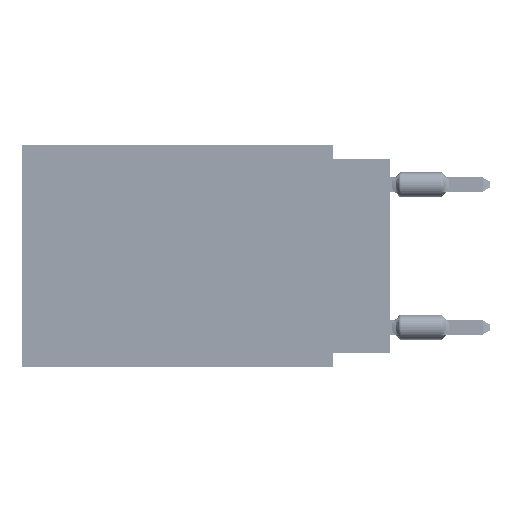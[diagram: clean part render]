
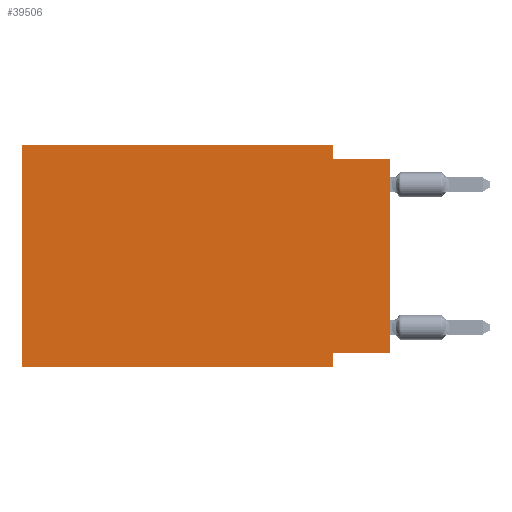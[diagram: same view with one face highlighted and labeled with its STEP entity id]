
A CAD part, left-side view. The second image highlights one B-rep face of the part: STEP entity #39506.
In plain terms, the highlighted planar face has unit normal (-1, 0, 0).
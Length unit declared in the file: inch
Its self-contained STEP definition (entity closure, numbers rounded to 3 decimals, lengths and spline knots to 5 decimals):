
#52 = ORIENTED_EDGE ( 'NONE', *, *, #19391, .F. ) ;
#125 = DIRECTION ( 'NONE',  ( 0., -1., 0. ) ) ;
#3661 = LINE ( 'NONE', #63159, #73262 ) ;
#3766 = CARTESIAN_POINT ( 'NONE',  ( 0., 0.1, -0.39 ) ) ;
#4742 = ORIENTED_EDGE ( 'NONE', *, *, #81338, .F. ) ;
#4808 = EDGE_LOOP ( 'NONE', ( #37551, #9426, #4742, #25082, #52, #56656, #25058, #45103 ) ) ;
#6551 = LINE ( 'NONE', #32664, #82076 ) ;
#8865 = VECTOR ( 'NONE', #70994, 39.37008 ) ;
#9426 = ORIENTED_EDGE ( 'NONE', *, *, #51864, .F. ) ;
#10950 = DIRECTION ( 'NONE',  ( 0., 0., -1. ) ) ;
#12824 = DIRECTION ( 'NONE',  ( 0., -1., 0. ) ) ;
#12857 = VECTOR ( 'NONE', #12824, 39.37008 ) ;
#14466 = VERTEX_POINT ( 'NONE', #17060 ) ;
#17060 = CARTESIAN_POINT ( 'NONE',  ( 0., 0.1, -0.025 ) ) ;
#17322 = CARTESIAN_POINT ( 'NONE',  ( 0., 0.1, -0.39 ) ) ;
#17599 = DIRECTION ( 'NONE',  ( 0., 0., -1. ) ) ;
#17921 = CARTESIAN_POINT ( 'NONE',  ( 0., 0.645, 0. ) ) ;
#17949 = VECTOR ( 'NONE', #71335, 39.37008 ) ;
#18405 = VERTEX_POINT ( 'NONE', #35603 ) ;
#19391 = EDGE_CURVE ( 'NONE', #18405, #36126, #3661, .T. ) ;
#21818 = FACE_OUTER_BOUND ( 'NONE', #4808, .T. ) ;
#22220 = CARTESIAN_POINT ( 'NONE',  ( 0., 0.645, 0. ) ) ;
#22279 = VECTOR ( 'NONE', #74169, 39.37008 ) ;
#23789 = DIRECTION ( 'NONE',  ( 1., 0., 0. ) ) ;
#24420 = CARTESIAN_POINT ( 'NONE',  ( 0., 0.1, 0. ) ) ;
#25058 = ORIENTED_EDGE ( 'NONE', *, *, #36834, .F. ) ;
#25082 = ORIENTED_EDGE ( 'NONE', *, *, #52332, .F. ) ;
#26493 = VECTOR ( 'NONE', #62937, 39.37008 ) ;
#31933 = CARTESIAN_POINT ( 'NONE',  ( 0., 0., -0.365 ) ) ;
#32664 = CARTESIAN_POINT ( 'NONE',  ( 0., 0.645, -0.39 ) ) ;
#32752 = VERTEX_POINT ( 'NONE', #67781 ) ;
#35136 = CARTESIAN_POINT ( 'NONE',  ( 0., 0.645, 0. ) ) ;
#35603 = CARTESIAN_POINT ( 'NONE',  ( 0., 0.645, -0.39 ) ) ;
#36126 = VERTEX_POINT ( 'NONE', #35136 ) ;
#36834 = EDGE_CURVE ( 'NONE', #72345, #54235, #74851, .T. ) ;
#37551 = ORIENTED_EDGE ( 'NONE', *, *, #62501, .T. ) ;
#39090 = EDGE_CURVE ( 'NONE', #45189, #72345, #48071, .T. ) ;
#39506 = ADVANCED_FACE ( 'NONE', ( #21818 ), #47973, .F. ) ;
#44523 = EDGE_CURVE ( 'NONE', #18405, #54235, #6551, .T. ) ;
#45103 = ORIENTED_EDGE ( 'NONE', *, *, #39090, .F. ) ;
#45189 = VERTEX_POINT ( 'NONE', #31933 ) ;
#45321 = LINE ( 'NONE', #17921, #8865 ) ;
#47973 = PLANE ( 'NONE',  #77065 ) ;
#48071 = LINE ( 'NONE', #68587, #22279 ) ;
#50905 = CARTESIAN_POINT ( 'NONE',  ( 0., 0., 0. ) ) ;
#51327 = LINE ( 'NONE', #50905, #26493 ) ;
#51374 = VERTEX_POINT ( 'NONE', #73970 ) ;
#51864 = EDGE_CURVE ( 'NONE', #14466, #32752, #56270, .T. ) ;
#52332 = EDGE_CURVE ( 'NONE', #36126, #51374, #45321, .T. ) ;
#54235 = VERTEX_POINT ( 'NONE', #17322 ) ;
#56270 = LINE ( 'NONE', #65542, #12857 ) ;
#56656 = ORIENTED_EDGE ( 'NONE', *, *, #44523, .T. ) ;
#61477 = DIRECTION ( 'NONE',  ( 0., 0., 1. ) ) ;
#62501 = EDGE_CURVE ( 'NONE', #45189, #32752, #51327, .T. ) ;
#62937 = DIRECTION ( 'NONE',  ( 0., 0., 1. ) ) ;
#63159 = CARTESIAN_POINT ( 'NONE',  ( 0., 0.645, 0. ) ) ;
#65542 = CARTESIAN_POINT ( 'NONE',  ( 0., 0., -0.025 ) ) ;
#67781 = CARTESIAN_POINT ( 'NONE',  ( 0., 0., -0.025 ) ) ;
#68587 = CARTESIAN_POINT ( 'NONE',  ( 0., 0., -0.365 ) ) ;
#70241 = LINE ( 'NONE', #24420, #75218 ) ;
#70994 = DIRECTION ( 'NONE',  ( 0., -1., 0. ) ) ;
#71335 = DIRECTION ( 'NONE',  ( 0., 0., -1. ) ) ;
#72345 = VERTEX_POINT ( 'NONE', #74001 ) ;
#73262 = VECTOR ( 'NONE', #61477, 39.37008 ) ;
#73970 = CARTESIAN_POINT ( 'NONE',  ( 0., 0.1, 0. ) ) ;
#74001 = CARTESIAN_POINT ( 'NONE',  ( 0., 0.1, -0.365 ) ) ;
#74169 = DIRECTION ( 'NONE',  ( 0., 1., 0. ) ) ;
#74851 = LINE ( 'NONE', #3766, #17949 ) ;
#75218 = VECTOR ( 'NONE', #17599, 39.37008 ) ;
#77065 = AXIS2_PLACEMENT_3D ( 'NONE', #22220, #23789, #10950 ) ;
#81338 = EDGE_CURVE ( 'NONE', #51374, #14466, #70241, .T. ) ;
#82076 = VECTOR ( 'NONE', #125, 39.37008 ) ;
